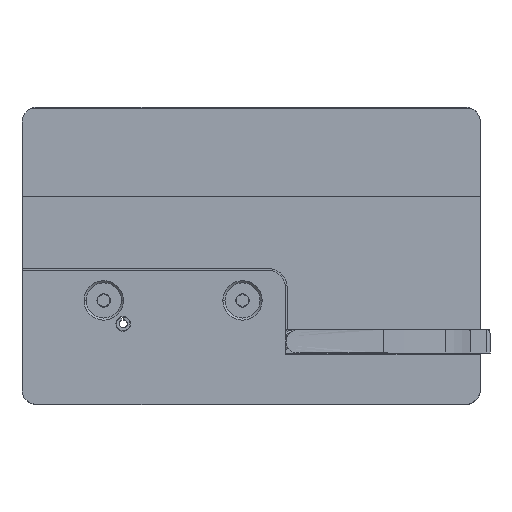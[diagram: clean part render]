
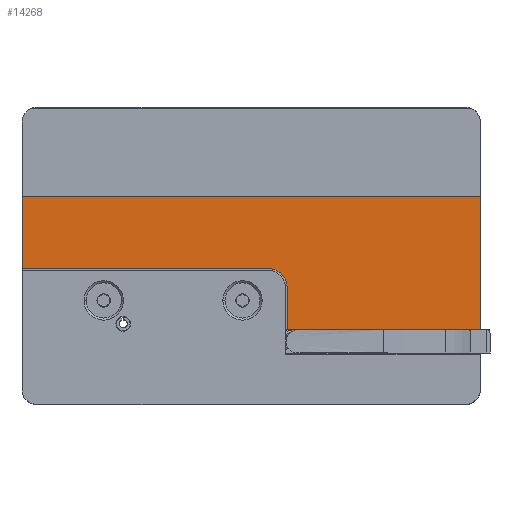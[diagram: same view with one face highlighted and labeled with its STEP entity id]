
A CAD part, top view. The second image highlights one B-rep face of the part: STEP entity #14268.
In plain terms, the highlighted face is planar.
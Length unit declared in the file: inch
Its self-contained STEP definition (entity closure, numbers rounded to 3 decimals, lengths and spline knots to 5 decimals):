
#265 = DIRECTION ( 'NONE',  ( 1., 0., 0. ) ) ;
#551 = EDGE_CURVE ( 'NONE', #1826, #10571, #15135, .T. ) ;
#631 = VERTEX_POINT ( 'NONE', #20141 ) ;
#710 = VERTEX_POINT ( 'NONE', #1774 ) ;
#1201 = DIRECTION ( 'NONE',  ( 0., 0., -1. ) ) ;
#1774 = CARTESIAN_POINT ( 'NONE',  ( -0.47, 1.03268, 0.125 ) ) ;
#1826 = VERTEX_POINT ( 'NONE', #7680 ) ;
#2024 = DIRECTION ( 'NONE',  ( 0., 1., 0. ) ) ;
#2204 = EDGE_CURVE ( 'NONE', #17065, #11586, #4663, .T. ) ;
#2389 = LINE ( 'NONE', #14279, #11090 ) ;
#2494 = DIRECTION ( 'NONE',  ( -1., 0., 0. ) ) ;
#2617 = ORIENTED_EDGE ( 'NONE', *, *, #20249, .T. ) ;
#2722 = CARTESIAN_POINT ( 'NONE',  ( -0.47, 0.54687, -1.175 ) ) ;
#3290 = CARTESIAN_POINT ( 'NONE',  ( -0.47, 0.42187, -1.175 ) ) ;
#3565 = ORIENTED_EDGE ( 'NONE', *, *, #17990, .T. ) ;
#4053 = AXIS2_PLACEMENT_3D ( 'NONE', #16317, #2494, #5932 ) ;
#4599 = EDGE_CURVE ( 'NONE', #710, #16467, #20979, .T. ) ;
#4663 = LINE ( 'NONE', #2722, #10788 ) ;
#5527 = DIRECTION ( 'NONE',  ( 0., 0., 1. ) ) ;
#5932 = DIRECTION ( 'NONE',  ( 0., 0., 1. ) ) ;
#6512 = CARTESIAN_POINT ( 'NONE',  ( -0.47, 0.54687, -2.95894 ) ) ;
#7090 = LINE ( 'NONE', #18717, #18005 ) ;
#7419 = DIRECTION ( 'NONE',  ( 0., 1., 0. ) ) ;
#7523 = CARTESIAN_POINT ( 'NONE',  ( -0.47, 1.03268, -2.95894 ) ) ;
#7680 = CARTESIAN_POINT ( 'NONE',  ( -0.47, 0.54687, -1.3 ) ) ;
#8756 = CARTESIAN_POINT ( 'NONE',  ( -0.47, 1.03268, 0.125 ) ) ;
#8771 = CARTESIAN_POINT ( 'NONE',  ( -0.47, 1.03268, -2.55894 ) ) ;
#9314 = VECTOR ( 'NONE', #2024, 39.37008 ) ;
#10571 = VERTEX_POINT ( 'NONE', #6512 ) ;
#10788 = VECTOR ( 'NONE', #20176, 39.37008 ) ;
#11090 = VECTOR ( 'NONE', #7419, 39.37008 ) ;
#11103 = CARTESIAN_POINT ( 'NONE',  ( -0.47, 0.42187, -1.3 ) ) ;
#11586 = VERTEX_POINT ( 'NONE', #18206 ) ;
#12095 = LINE ( 'NONE', #8756, #9314 ) ;
#12456 = PLANE ( 'NONE',  #4053 ) ;
#14028 = DIRECTION ( 'NONE',  ( 0., 0., -1. ) ) ;
#14038 = VECTOR ( 'NONE', #1201, 39.37008 ) ;
#14268 = ADVANCED_FACE ( 'NONE', ( #18021 ), #12456, .T. ) ;
#14279 = CARTESIAN_POINT ( 'NONE',  ( -0.47, -0.02313, -2.95894 ) ) ;
#15135 = LINE ( 'NONE', #17068, #14038 ) ;
#15160 = ORIENTED_EDGE ( 'NONE', *, *, #4599, .T. ) ;
#15313 = DIRECTION ( 'NONE',  ( 0., 0., 1. ) ) ;
#15328 = ORIENTED_EDGE ( 'NONE', *, *, #17650, .T. ) ;
#16317 = CARTESIAN_POINT ( 'NONE',  ( -0.47, 0., 0. ) ) ;
#16467 = VERTEX_POINT ( 'NONE', #7523 ) ;
#17065 = VERTEX_POINT ( 'NONE', #3290 ) ;
#17068 = CARTESIAN_POINT ( 'NONE',  ( -0.47, 0.54687, 0. ) ) ;
#17200 = EDGE_LOOP ( 'NONE', ( #20841, #15328, #18248, #3565, #2617, #15160, #20621 ) ) ;
#17650 = EDGE_CURVE ( 'NONE', #1826, #17065, #18266, .T. ) ;
#17990 = EDGE_CURVE ( 'NONE', #11586, #631, #7090, .T. ) ;
#18005 = VECTOR ( 'NONE', #15313, 39.37008 ) ;
#18021 = FACE_OUTER_BOUND ( 'NONE', #17200, .T. ) ;
#18206 = CARTESIAN_POINT ( 'NONE',  ( -0.47, 0.13829, -1.175 ) ) ;
#18248 = ORIENTED_EDGE ( 'NONE', *, *, #2204, .T. ) ;
#18264 = EDGE_CURVE ( 'NONE', #10571, #16467, #2389, .T. ) ;
#18266 = CIRCLE ( 'NONE', #21195, 0.125 ) ;
#18717 = CARTESIAN_POINT ( 'NONE',  ( -0.47, 0.13829, 0.125 ) ) ;
#20141 = CARTESIAN_POINT ( 'NONE',  ( -0.47, 0.13829, 0.125 ) ) ;
#20176 = DIRECTION ( 'NONE',  ( 0., -1., 0. ) ) ;
#20249 = EDGE_CURVE ( 'NONE', #631, #710, #12095, .T. ) ;
#20621 = ORIENTED_EDGE ( 'NONE', *, *, #18264, .F. ) ;
#20841 = ORIENTED_EDGE ( 'NONE', *, *, #551, .F. ) ;
#20979 = LINE ( 'NONE', #8771, #21410 ) ;
#21195 = AXIS2_PLACEMENT_3D ( 'NONE', #11103, #265, #5527 ) ;
#21410 = VECTOR ( 'NONE', #14028, 39.37008 ) ;
